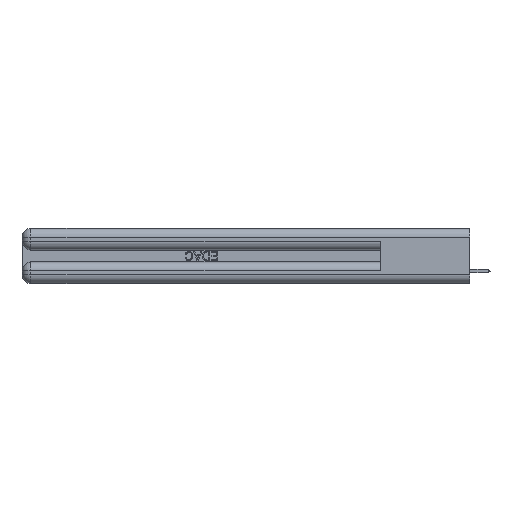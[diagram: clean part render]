
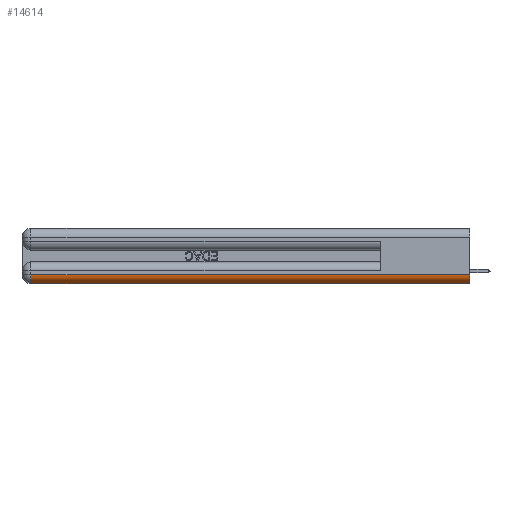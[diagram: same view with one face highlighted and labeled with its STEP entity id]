
A CAD part, left-side view. The second image highlights one B-rep face of the part: STEP entity #14614.
In plain terms, the highlighted cylindrical face has radius 1.524 mm (diameter 3.048 mm), a partial arc.
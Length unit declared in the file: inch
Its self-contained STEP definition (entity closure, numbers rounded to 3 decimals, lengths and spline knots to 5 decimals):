
#954 = AXIS2_PLACEMENT_3D ( 'NONE', #42721, #23861, #31865 ) ;
#2596 = AXIS2_PLACEMENT_3D ( 'NONE', #17442, #38015, #24940 ) ;
#3424 = DIRECTION ( 'NONE',  ( 0., 0., 1. ) ) ;
#3923 = EDGE_CURVE ( 'NONE', #32323, #27241, #43648, .T. ) ;
#3961 = EDGE_LOOP ( 'NONE', ( #17996, #33494, #15893, #34064 ) ) ;
#4677 = CARTESIAN_POINT ( 'NONE',  ( 0.06, 0., 0. ) ) ;
#4823 = FACE_OUTER_BOUND ( 'NONE', #3961, .T. ) ;
#6623 = EDGE_CURVE ( 'NONE', #30850, #19065, #29078, .T. ) ;
#6799 = DIRECTION ( 'NONE',  ( 0., -1., 0. ) ) ;
#7793 = CIRCLE ( 'NONE', #954, 0.06 ) ;
#9912 = VECTOR ( 'NONE', #28029, 39.37008 ) ;
#13709 = CARTESIAN_POINT ( 'NONE',  ( 0., 0., 0.06 ) ) ;
#13772 = EDGE_CURVE ( 'NONE', #19065, #32323, #7793, .T. ) ;
#14614 = ADVANCED_FACE ( 'NONE', ( #4823 ), #30013, .T. ) ;
#15893 = ORIENTED_EDGE ( 'NONE', *, *, #31470, .F. ) ;
#17442 = CARTESIAN_POINT ( 'NONE',  ( 0.06, 0., 0.06 ) ) ;
#17553 = CARTESIAN_POINT ( 'NONE',  ( 0., 2.94, 0.06 ) ) ;
#17992 = DIRECTION ( 'NONE',  ( 0., 1., 0. ) ) ;
#17996 = ORIENTED_EDGE ( 'NONE', *, *, #13772, .F. ) ;
#19065 = VERTEX_POINT ( 'NONE', #13709 ) ;
#23861 = DIRECTION ( 'NONE',  ( 0., -1., 0. ) ) ;
#24828 = CIRCLE ( 'NONE', #45545, 0.06 ) ;
#24940 = DIRECTION ( 'NONE',  ( 0., 0., 1. ) ) ;
#25360 = CARTESIAN_POINT ( 'NONE',  ( 0., 0., 0.06 ) ) ;
#27241 = VERTEX_POINT ( 'NONE', #33360 ) ;
#28029 = DIRECTION ( 'NONE',  ( 0., 1., 0. ) ) ;
#29078 = LINE ( 'NONE', #25360, #47341 ) ;
#30013 = CYLINDRICAL_SURFACE ( 'NONE', #2596, 0.06 ) ;
#30850 = VERTEX_POINT ( 'NONE', #17553 ) ;
#31470 = EDGE_CURVE ( 'NONE', #27241, #30850, #24828, .T. ) ;
#31865 = DIRECTION ( 'NONE',  ( 0., 0., 1. ) ) ;
#32323 = VERTEX_POINT ( 'NONE', #4677 ) ;
#33360 = CARTESIAN_POINT ( 'NONE',  ( 0.06, 2.94, 0. ) ) ;
#33494 = ORIENTED_EDGE ( 'NONE', *, *, #6623, .F. ) ;
#34064 = ORIENTED_EDGE ( 'NONE', *, *, #3923, .F. ) ;
#35194 = CARTESIAN_POINT ( 'NONE',  ( 0.06, 3., 0. ) ) ;
#38015 = DIRECTION ( 'NONE',  ( 0., 1., 0. ) ) ;
#42721 = CARTESIAN_POINT ( 'NONE',  ( 0.06, 0., 0.06 ) ) ;
#43648 = LINE ( 'NONE', #35194, #9912 ) ;
#43709 = CARTESIAN_POINT ( 'NONE',  ( 0.06, 2.94, 0.06 ) ) ;
#45545 = AXIS2_PLACEMENT_3D ( 'NONE', #43709, #17992, #3424 ) ;
#47341 = VECTOR ( 'NONE', #6799, 39.37008 ) ;
